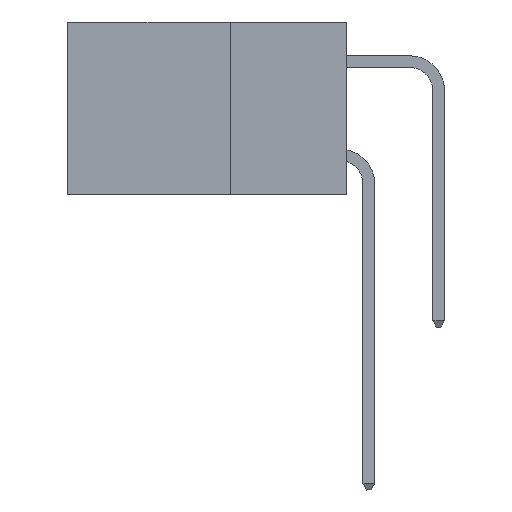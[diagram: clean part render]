
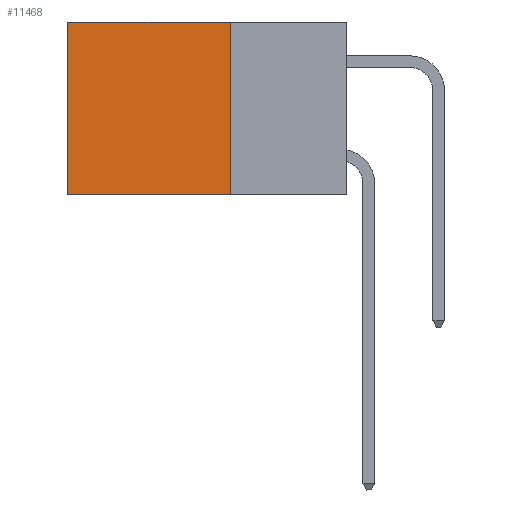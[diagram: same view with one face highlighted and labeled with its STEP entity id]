
A CAD part, left-side view. The second image highlights one B-rep face of the part: STEP entity #11468.
In plain terms, the highlighted planar face has unit normal (-1, 0, 0).
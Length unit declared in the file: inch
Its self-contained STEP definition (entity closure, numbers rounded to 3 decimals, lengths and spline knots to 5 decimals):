
#1640 = EDGE_LOOP ( 'NONE', ( #20624, #26460, #15932, #5278 ) ) ;
#3289 = VECTOR ( 'NONE', #9025, 39.37008 ) ;
#4718 = AXIS2_PLACEMENT_3D ( 'NONE', #24964, #25062, #16774 ) ;
#5248 = LINE ( 'NONE', #25555, #3289 ) ;
#5278 = ORIENTED_EDGE ( 'NONE', *, *, #9030, .T. ) ;
#5475 = CARTESIAN_POINT ( 'NONE',  ( 0.2875, 0.25, 0. ) ) ;
#6019 = DIRECTION ( 'NONE',  ( 0., 1., 0. ) ) ;
#6644 = VERTEX_POINT ( 'NONE', #5475 ) ;
#7619 = EDGE_CURVE ( 'NONE', #22811, #10139, #9957, .T. ) ;
#8749 = PLANE ( 'NONE',  #4718 ) ;
#9025 = DIRECTION ( 'NONE',  ( 0., 1., 0. ) ) ;
#9030 = EDGE_CURVE ( 'NONE', #6644, #22811, #9568, .T. ) ;
#9568 = LINE ( 'NONE', #20158, #24156 ) ;
#9957 = LINE ( 'NONE', #11826, #11608 ) ;
#10102 = VECTOR ( 'NONE', #17400, 39.37008 ) ;
#10139 = VERTEX_POINT ( 'NONE', #14064 ) ;
#11468 = ADVANCED_FACE ( 'NONE', ( #11892 ), #8749, .F. ) ;
#11565 = CARTESIAN_POINT ( 'NONE',  ( 0.2875, 0.6, 0. ) ) ;
#11608 = VECTOR ( 'NONE', #13880, 39.37008 ) ;
#11826 = CARTESIAN_POINT ( 'NONE',  ( 0.2875, 0.6, 0. ) ) ;
#11892 = FACE_OUTER_BOUND ( 'NONE', #1640, .T. ) ;
#13880 = DIRECTION ( 'NONE',  ( 0., 0., -1. ) ) ;
#14064 = CARTESIAN_POINT ( 'NONE',  ( 0.2875, 0.6, -0.37 ) ) ;
#14381 = EDGE_CURVE ( 'NONE', #6644, #16577, #16556, .T. ) ;
#15538 = EDGE_CURVE ( 'NONE', #16577, #10139, #5248, .T. ) ;
#15932 = ORIENTED_EDGE ( 'NONE', *, *, #14381, .F. ) ;
#16556 = LINE ( 'NONE', #23900, #10102 ) ;
#16577 = VERTEX_POINT ( 'NONE', #23240 ) ;
#16774 = DIRECTION ( 'NONE',  ( 0., 0., -1. ) ) ;
#17400 = DIRECTION ( 'NONE',  ( 0., 0., -1. ) ) ;
#20158 = CARTESIAN_POINT ( 'NONE',  ( 0.2875, 0.25, 0. ) ) ;
#20624 = ORIENTED_EDGE ( 'NONE', *, *, #7619, .T. ) ;
#22811 = VERTEX_POINT ( 'NONE', #11565 ) ;
#23240 = CARTESIAN_POINT ( 'NONE',  ( 0.2875, 0.25, -0.37 ) ) ;
#23900 = CARTESIAN_POINT ( 'NONE',  ( 0.2875, 0.25, 0. ) ) ;
#24156 = VECTOR ( 'NONE', #6019, 39.37008 ) ;
#24964 = CARTESIAN_POINT ( 'NONE',  ( 0.2875, 0.25, 0. ) ) ;
#25062 = DIRECTION ( 'NONE',  ( 1., 0., 0. ) ) ;
#25555 = CARTESIAN_POINT ( 'NONE',  ( 0.2875, 0.25, -0.37 ) ) ;
#26460 = ORIENTED_EDGE ( 'NONE', *, *, #15538, .F. ) ;
